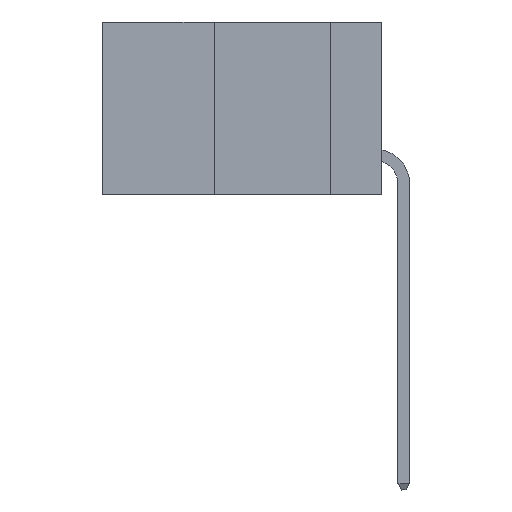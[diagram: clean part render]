
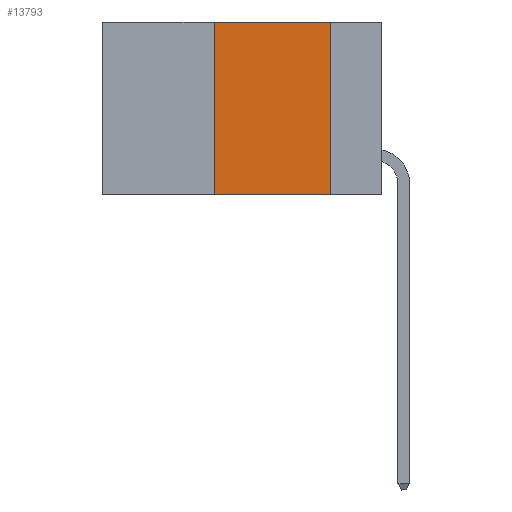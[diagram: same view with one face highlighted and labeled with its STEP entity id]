
A CAD part, left-side view. The second image highlights one B-rep face of the part: STEP entity #13793.
In plain terms, the highlighted planar face has unit normal (-1, 0, 0).
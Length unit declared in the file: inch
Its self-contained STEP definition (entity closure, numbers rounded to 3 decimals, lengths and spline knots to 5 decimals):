
#75 = EDGE_LOOP ( 'NONE', ( #3177, #11280, #8331, #1242 ) ) ;
#408 = VECTOR ( 'NONE', #3786, 39.37008 ) ;
#813 = CARTESIAN_POINT ( 'NONE',  ( 0., 0.36, -0.37 ) ) ;
#1242 = ORIENTED_EDGE ( 'NONE', *, *, #13859, .T. ) ;
#1584 = LINE ( 'NONE', #15744, #13299 ) ;
#2036 = DIRECTION ( 'NONE',  ( 0., 0., 1. ) ) ;
#2062 = CARTESIAN_POINT ( 'NONE',  ( 0., 0.11, 0. ) ) ;
#2078 = VERTEX_POINT ( 'NONE', #2062 ) ;
#2569 = LINE ( 'NONE', #13043, #4441 ) ;
#2759 = CARTESIAN_POINT ( 'NONE',  ( 0., 0.6, -0.37 ) ) ;
#3177 = ORIENTED_EDGE ( 'NONE', *, *, #11211, .F. ) ;
#3786 = DIRECTION ( 'NONE',  ( 0., -1., 0. ) ) ;
#4284 = DIRECTION ( 'NONE',  ( 0., -1., 0. ) ) ;
#4441 = VECTOR ( 'NONE', #4876, 39.37008 ) ;
#4765 = VECTOR ( 'NONE', #4284, 39.37008 ) ;
#4876 = DIRECTION ( 'NONE',  ( 0., 0., -1. ) ) ;
#4942 = EDGE_CURVE ( 'NONE', #8319, #2078, #6551, .T. ) ;
#5347 = CARTESIAN_POINT ( 'NONE',  ( 0., 0.6, 0. ) ) ;
#6551 = LINE ( 'NONE', #7736, #408 ) ;
#7736 = CARTESIAN_POINT ( 'NONE',  ( 0., 0.6, 0. ) ) ;
#8319 = VERTEX_POINT ( 'NONE', #17505 ) ;
#8331 = ORIENTED_EDGE ( 'NONE', *, *, #14149, .F. ) ;
#8881 = AXIS2_PLACEMENT_3D ( 'NONE', #5347, #13466, #10837 ) ;
#10356 = VERTEX_POINT ( 'NONE', #16919 ) ;
#10837 = DIRECTION ( 'NONE',  ( 0., 0., -1. ) ) ;
#11211 = EDGE_CURVE ( 'NONE', #2078, #10356, #2569, .T. ) ;
#11280 = ORIENTED_EDGE ( 'NONE', *, *, #4942, .F. ) ;
#11468 = VERTEX_POINT ( 'NONE', #813 ) ;
#12022 = LINE ( 'NONE', #2759, #4765 ) ;
#12157 = PLANE ( 'NONE',  #8881 ) ;
#13043 = CARTESIAN_POINT ( 'NONE',  ( 0., 0.11, 0. ) ) ;
#13299 = VECTOR ( 'NONE', #2036, 39.37008 ) ;
#13466 = DIRECTION ( 'NONE',  ( 1., 0., 0. ) ) ;
#13793 = ADVANCED_FACE ( 'NONE', ( #17095 ), #12157, .F. ) ;
#13859 = EDGE_CURVE ( 'NONE', #11468, #10356, #12022, .T. ) ;
#14149 = EDGE_CURVE ( 'NONE', #11468, #8319, #1584, .T. ) ;
#15744 = CARTESIAN_POINT ( 'NONE',  ( 0., 0.36, 0. ) ) ;
#16919 = CARTESIAN_POINT ( 'NONE',  ( 0., 0.11, -0.37 ) ) ;
#17095 = FACE_OUTER_BOUND ( 'NONE', #75, .T. ) ;
#17505 = CARTESIAN_POINT ( 'NONE',  ( 0., 0.36, 0. ) ) ;
